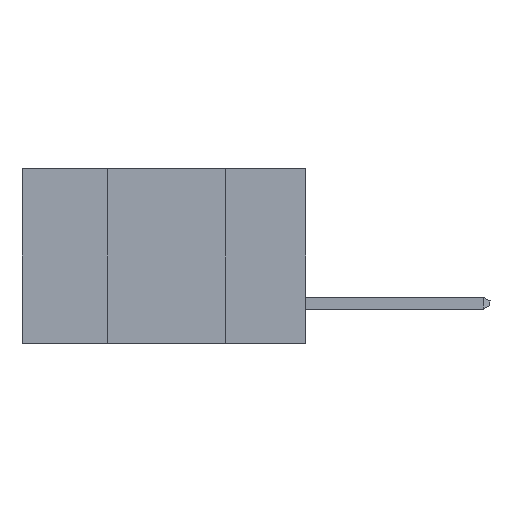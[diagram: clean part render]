
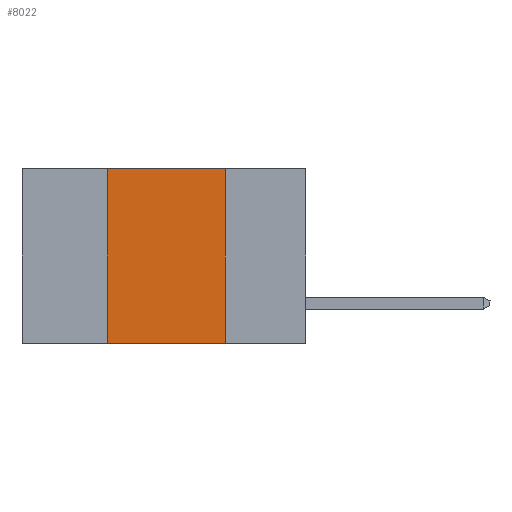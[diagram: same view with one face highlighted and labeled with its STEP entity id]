
A CAD part, left-side view. The second image highlights one B-rep face of the part: STEP entity #8022.
In plain terms, the highlighted planar face has unit normal (-1, 0, 0).
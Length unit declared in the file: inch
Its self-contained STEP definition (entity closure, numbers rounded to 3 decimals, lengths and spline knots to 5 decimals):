
#152 = LINE ( 'NONE', #7240, #10006 ) ;
#210 = EDGE_CURVE ( 'NONE', #7793, #7862, #9550, .T. ) ;
#425 = VECTOR ( 'NONE', #9878, 39.37008 ) ;
#921 = CARTESIAN_POINT ( 'NONE',  ( 0., 0.17, -0.37 ) ) ;
#2022 = DIRECTION ( 'NONE',  ( 0., 0., -1. ) ) ;
#2426 = VERTEX_POINT ( 'NONE', #11647 ) ;
#2683 = CARTESIAN_POINT ( 'NONE',  ( 0., 0.42, 0. ) ) ;
#2762 = EDGE_CURVE ( 'NONE', #2995, #2426, #10789, .T. ) ;
#2855 = EDGE_CURVE ( 'NONE', #7793, #2426, #12020, .T. ) ;
#2995 = VERTEX_POINT ( 'NONE', #4824 ) ;
#3008 = DIRECTION ( 'NONE',  ( 0., -1., 0. ) ) ;
#3590 = EDGE_CURVE ( 'NONE', #7862, #2995, #152, .T. ) ;
#3619 = ORIENTED_EDGE ( 'NONE', *, *, #2762, .F. ) ;
#3843 = ORIENTED_EDGE ( 'NONE', *, *, #3590, .F. ) ;
#4824 = CARTESIAN_POINT ( 'NONE',  ( 0., 0.17, 0. ) ) ;
#4982 = FACE_OUTER_BOUND ( 'NONE', #12449, .T. ) ;
#6201 = CARTESIAN_POINT ( 'NONE',  ( 0., 0.6, -0.37 ) ) ;
#6741 = ORIENTED_EDGE ( 'NONE', *, *, #210, .F. ) ;
#6845 = PLANE ( 'NONE',  #6891 ) ;
#6891 = AXIS2_PLACEMENT_3D ( 'NONE', #11716, #8978, #2022 ) ;
#7240 = CARTESIAN_POINT ( 'NONE',  ( 0., 0.6, 0. ) ) ;
#7793 = VERTEX_POINT ( 'NONE', #8340 ) ;
#7862 = VERTEX_POINT ( 'NONE', #2683 ) ;
#8022 = ADVANCED_FACE ( 'NONE', ( #4982 ), #6845, .F. ) ;
#8340 = CARTESIAN_POINT ( 'NONE',  ( 0., 0.42, -0.37 ) ) ;
#8937 = ORIENTED_EDGE ( 'NONE', *, *, #2855, .T. ) ;
#8978 = DIRECTION ( 'NONE',  ( 1., 0., 0. ) ) ;
#9146 = VECTOR ( 'NONE', #10629, 39.37008 ) ;
#9550 = LINE ( 'NONE', #10505, #9146 ) ;
#9878 = DIRECTION ( 'NONE',  ( 0., 0., -1. ) ) ;
#9962 = VECTOR ( 'NONE', #3008, 39.37008 ) ;
#10006 = VECTOR ( 'NONE', #12034, 39.37008 ) ;
#10505 = CARTESIAN_POINT ( 'NONE',  ( 0., 0.42, -0.37 ) ) ;
#10629 = DIRECTION ( 'NONE',  ( 0., 0., 1. ) ) ;
#10789 = LINE ( 'NONE', #921, #425 ) ;
#11647 = CARTESIAN_POINT ( 'NONE',  ( 0., 0.17, -0.37 ) ) ;
#11716 = CARTESIAN_POINT ( 'NONE',  ( 0., 0.6, 0. ) ) ;
#12020 = LINE ( 'NONE', #6201, #9962 ) ;
#12034 = DIRECTION ( 'NONE',  ( 0., -1., 0. ) ) ;
#12449 = EDGE_LOOP ( 'NONE', ( #3619, #3843, #6741, #8937 ) ) ;
